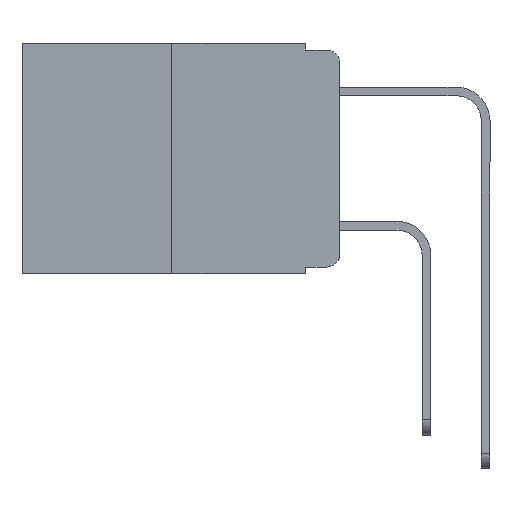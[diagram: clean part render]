
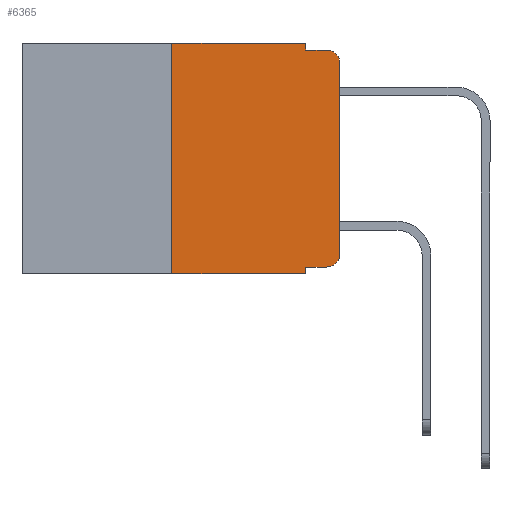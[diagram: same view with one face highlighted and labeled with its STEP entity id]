
A CAD part, left-side view. The second image highlights one B-rep face of the part: STEP entity #6365.
In plain terms, the highlighted planar face has unit normal (-1, 0, 0).
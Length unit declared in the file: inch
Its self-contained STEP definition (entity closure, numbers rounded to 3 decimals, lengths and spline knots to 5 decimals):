
#34 = VECTOR ( 'NONE', #7087, 39.37008 ) ;
#117 = CARTESIAN_POINT ( 'NONE',  ( 0., 0.051, 0. ) ) ;
#902 = VERTEX_POINT ( 'NONE', #9737 ) ;
#1046 = CARTESIAN_POINT ( 'NONE',  ( 0., 0., -0.03 ) ) ;
#1144 = CARTESIAN_POINT ( 'NONE',  ( 0., 0.473, -0.343 ) ) ;
#1264 = VERTEX_POINT ( 'NONE', #4941 ) ;
#1372 = CIRCLE ( 'NONE', #3072, 0.02 ) ;
#1832 = EDGE_CURVE ( 'NONE', #10589, #10627, #8958, .T. ) ;
#1923 = VECTOR ( 'NONE', #9174, 39.37008 ) ;
#1932 = ORIENTED_EDGE ( 'NONE', *, *, #1832, .T. ) ;
#1954 = ORIENTED_EDGE ( 'NONE', *, *, #3861, .T. ) ;
#2103 = ORIENTED_EDGE ( 'NONE', *, *, #8759, .F. ) ;
#2115 = ORIENTED_EDGE ( 'NONE', *, *, #5236, .F. ) ;
#2157 = DIRECTION ( 'NONE',  ( 0., 0., -1. ) ) ;
#2195 = ORIENTED_EDGE ( 'NONE', *, *, #8498, .F. ) ;
#2274 = ORIENTED_EDGE ( 'NONE', *, *, #2655, .F. ) ;
#2296 = ORIENTED_EDGE ( 'NONE', *, *, #2845, .T. ) ;
#2353 = ORIENTED_EDGE ( 'NONE', *, *, #10657, .F. ) ;
#2503 = ORIENTED_EDGE ( 'NONE', *, *, #8421, .T. ) ;
#2529 = ORIENTED_EDGE ( 'NONE', *, *, #9321, .T. ) ;
#2583 = VERTEX_POINT ( 'NONE', #6497 ) ;
#2625 = VECTOR ( 'NONE', #6458, 39.37008 ) ;
#2655 = EDGE_CURVE ( 'NONE', #902, #4013, #6786, .T. ) ;
#2684 = CARTESIAN_POINT ( 'NONE',  ( 0., 0.051, -0.01 ) ) ;
#2845 = EDGE_CURVE ( 'NONE', #902, #8987, #5316, .T. ) ;
#2977 = AXIS2_PLACEMENT_3D ( 'NONE', #4042, #7704, #2157 ) ;
#3008 = CARTESIAN_POINT ( 'NONE',  ( 0., 0.02, -0.333 ) ) ;
#3017 = VERTEX_POINT ( 'NONE', #3008 ) ;
#3072 = AXIS2_PLACEMENT_3D ( 'NONE', #9158, #4462, #9931 ) ;
#3375 = VECTOR ( 'NONE', #3456, 39.37008 ) ;
#3386 = AXIS2_PLACEMENT_3D ( 'NONE', #7936, #9470, #4814 ) ;
#3404 = CIRCLE ( 'NONE', #2977, 0.02 ) ;
#3456 = DIRECTION ( 'NONE',  ( 0., 0., -1. ) ) ;
#3861 = EDGE_CURVE ( 'NONE', #10627, #7596, #3404, .T. ) ;
#3875 = VERTEX_POINT ( 'NONE', #5100 ) ;
#4013 = VERTEX_POINT ( 'NONE', #5036 ) ;
#4030 = DIRECTION ( 'NONE',  ( 0., -1., 0. ) ) ;
#4042 = CARTESIAN_POINT ( 'NONE',  ( 0., 0.02, -0.03 ) ) ;
#4154 = DIRECTION ( 'NONE',  ( 0., 0., 1. ) ) ;
#4169 = LINE ( 'NONE', #117, #2625 ) ;
#4462 = DIRECTION ( 'NONE',  ( -1., 0., 0. ) ) ;
#4814 = DIRECTION ( 'NONE',  ( 0., 0., -1. ) ) ;
#4941 = CARTESIAN_POINT ( 'NONE',  ( 0., 0.051, -0.333 ) ) ;
#4945 = CARTESIAN_POINT ( 'NONE',  ( 0., 0.02, -0.01 ) ) ;
#5036 = CARTESIAN_POINT ( 'NONE',  ( 0., 0.25, 0. ) ) ;
#5100 = CARTESIAN_POINT ( 'NONE',  ( 0., 0.051, -0.01 ) ) ;
#5236 = EDGE_CURVE ( 'NONE', #2583, #3875, #5629, .T. ) ;
#5316 = LINE ( 'NONE', #1144, #34 ) ;
#5326 = DIRECTION ( 'NONE',  ( 0., -1., 0. ) ) ;
#5529 = VECTOR ( 'NONE', #5326, 39.37008 ) ;
#5556 = EDGE_LOOP ( 'NONE', ( #1932, #1954, #2103, #2115, #2195, #2274, #2296, #2353, #2503, #2529 ) ) ;
#5629 = LINE ( 'NONE', #9212, #3375 ) ;
#5893 = LINE ( 'NONE', #8099, #9747 ) ;
#6365 = ADVANCED_FACE ( 'NONE', ( #10881 ), #8716, .F. ) ;
#6458 = DIRECTION ( 'NONE',  ( 0., 0., -1. ) ) ;
#6497 = CARTESIAN_POINT ( 'NONE',  ( 0., 0.051, 0. ) ) ;
#6786 = LINE ( 'NONE', #10000, #1923 ) ;
#6909 = VECTOR ( 'NONE', #4154, 39.37008 ) ;
#7087 = DIRECTION ( 'NONE',  ( 0., -1., 0. ) ) ;
#7223 = CARTESIAN_POINT ( 'NONE',  ( 0., 0.051, -0.333 ) ) ;
#7310 = CARTESIAN_POINT ( 'NONE',  ( 0., 0., 0. ) ) ;
#7596 = VERTEX_POINT ( 'NONE', #4945 ) ;
#7704 = DIRECTION ( 'NONE',  ( -1., 0., 0. ) ) ;
#7936 = CARTESIAN_POINT ( 'NONE',  ( 0., 0.473, 0. ) ) ;
#8099 = CARTESIAN_POINT ( 'NONE',  ( 0., 0.473, 0. ) ) ;
#8421 = EDGE_CURVE ( 'NONE', #1264, #3017, #8913, .T. ) ;
#8498 = EDGE_CURVE ( 'NONE', #4013, #2583, #5893, .T. ) ;
#8641 = CARTESIAN_POINT ( 'NONE',  ( 0., 0., -0.313 ) ) ;
#8716 = PLANE ( 'NONE',  #3386 ) ;
#8740 = CARTESIAN_POINT ( 'NONE',  ( 0., 0.051, -0.343 ) ) ;
#8759 = EDGE_CURVE ( 'NONE', #3875, #7596, #9864, .T. ) ;
#8886 = DIRECTION ( 'NONE',  ( 0., -1., 0. ) ) ;
#8913 = LINE ( 'NONE', #7223, #10698 ) ;
#8958 = LINE ( 'NONE', #7310, #6909 ) ;
#8987 = VERTEX_POINT ( 'NONE', #8740 ) ;
#9158 = CARTESIAN_POINT ( 'NONE',  ( 0., 0.02, -0.313 ) ) ;
#9174 = DIRECTION ( 'NONE',  ( 0., 0., 1. ) ) ;
#9212 = CARTESIAN_POINT ( 'NONE',  ( 0., 0.051, 0. ) ) ;
#9321 = EDGE_CURVE ( 'NONE', #3017, #10589, #1372, .T. ) ;
#9470 = DIRECTION ( 'NONE',  ( 1., 0., 0. ) ) ;
#9737 = CARTESIAN_POINT ( 'NONE',  ( 0., 0.25, -0.343 ) ) ;
#9747 = VECTOR ( 'NONE', #8886, 39.37008 ) ;
#9864 = LINE ( 'NONE', #2684, #5529 ) ;
#9931 = DIRECTION ( 'NONE',  ( 0., 0., -1. ) ) ;
#10000 = CARTESIAN_POINT ( 'NONE',  ( 0., 0.25, 0. ) ) ;
#10589 = VERTEX_POINT ( 'NONE', #8641 ) ;
#10627 = VERTEX_POINT ( 'NONE', #1046 ) ;
#10657 = EDGE_CURVE ( 'NONE', #1264, #8987, #4169, .T. ) ;
#10698 = VECTOR ( 'NONE', #4030, 39.37008 ) ;
#10881 = FACE_OUTER_BOUND ( 'NONE', #5556, .T. ) ;
